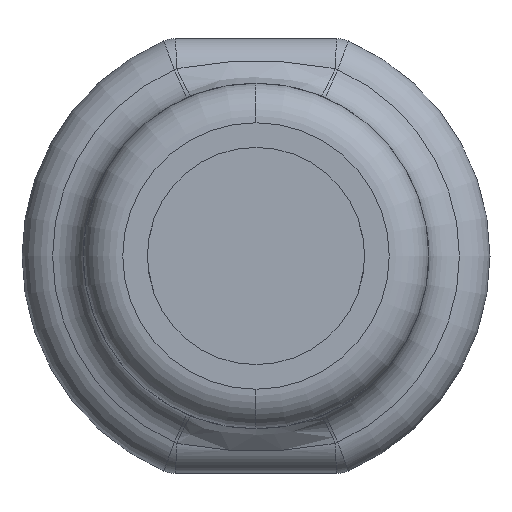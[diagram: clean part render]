
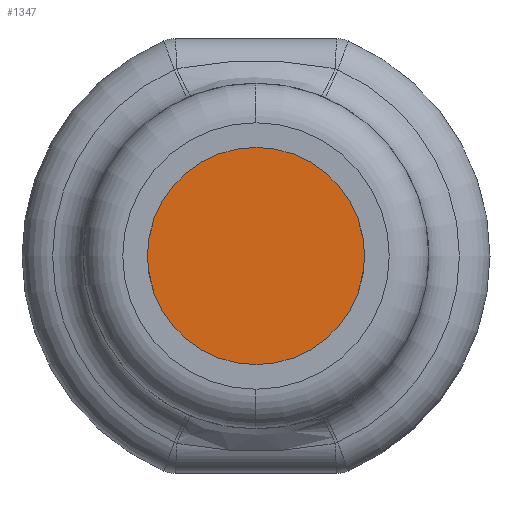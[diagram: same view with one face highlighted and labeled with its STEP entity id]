
A CAD part, left-side view. The second image highlights one B-rep face of the part: STEP entity #1347.
In plain terms, the highlighted planar face has unit normal (-1, 0, 0).
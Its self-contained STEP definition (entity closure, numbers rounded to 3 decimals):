
#112 = EDGE_LOOP ( 'NONE', ( #3144, #3269 ) ) ;
#365 = AXIS2_PLACEMENT_3D ( 'NONE', #1950, #2994, #1998 ) ;
#483 = VERTEX_POINT ( 'NONE', #3050 ) ;
#532 = CIRCLE ( 'NONE', #2025, 11. ) ;
#688 = CARTESIAN_POINT ( 'NONE',  ( -259.382, 25.482, -11.277 ) ) ;
#874 = DIRECTION ( 'NONE',  ( 0., 0., 1. ) ) ;
#1155 = CARTESIAN_POINT ( 'NONE',  ( -259.382, 25.482, -0.277 ) ) ;
#1347 = ADVANCED_FACE ( 'NONE', ( #1906 ), #3236, .T. ) ;
#1681 = EDGE_CURVE ( 'NONE', #2009, #483, #1873, .T. ) ;
#1810 = AXIS2_PLACEMENT_3D ( 'NONE', #1874, #2664, #874 ) ;
#1873 = CIRCLE ( 'NONE', #365, 11. ) ;
#1874 = CARTESIAN_POINT ( 'NONE',  ( -259.382, 25.482, -0.277 ) ) ;
#1896 = DIRECTION ( 'NONE',  ( -1., 0., 0. ) ) ;
#1906 = FACE_OUTER_BOUND ( 'NONE', #112, .T. ) ;
#1950 = CARTESIAN_POINT ( 'NONE',  ( -259.382, 25.482, -0.277 ) ) ;
#1998 = DIRECTION ( 'NONE',  ( 0., 0., 1. ) ) ;
#2009 = VERTEX_POINT ( 'NONE', #688 ) ;
#2025 = AXIS2_PLACEMENT_3D ( 'NONE', #1155, #1896, #2213 ) ;
#2213 = DIRECTION ( 'NONE',  ( 0., 0., 1. ) ) ;
#2664 = DIRECTION ( 'NONE',  ( -1., 0., 0. ) ) ;
#2994 = DIRECTION ( 'NONE',  ( -1., 0., 0. ) ) ;
#3050 = CARTESIAN_POINT ( 'NONE',  ( -259.382, 25.482, 10.723 ) ) ;
#3144 = ORIENTED_EDGE ( 'NONE', *, *, #3202, .T. ) ;
#3202 = EDGE_CURVE ( 'NONE', #483, #2009, #532, .T. ) ;
#3236 = PLANE ( 'NONE',  #1810 ) ;
#3269 = ORIENTED_EDGE ( 'NONE', *, *, #1681, .T. ) ;
